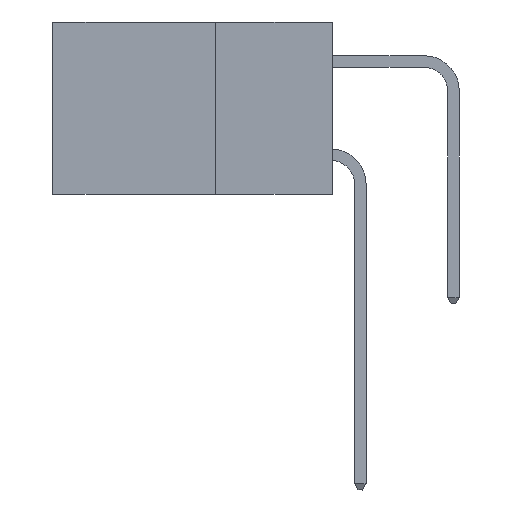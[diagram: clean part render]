
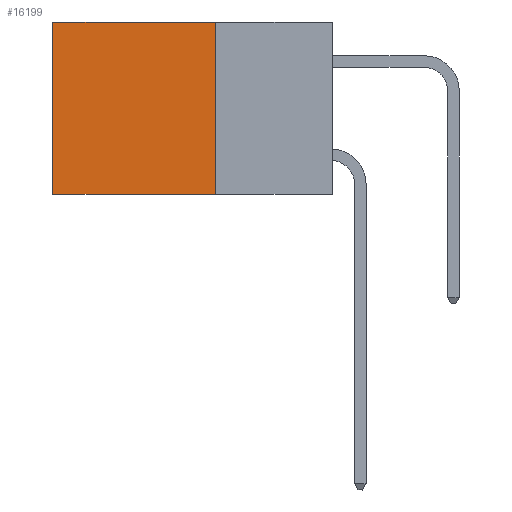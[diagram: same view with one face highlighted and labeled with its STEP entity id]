
A CAD part, left-side view. The second image highlights one B-rep face of the part: STEP entity #16199.
In plain terms, the highlighted planar face has unit normal (-1, 0, 0).
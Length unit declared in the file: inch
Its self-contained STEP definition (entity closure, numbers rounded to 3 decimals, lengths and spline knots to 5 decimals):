
#566 = EDGE_LOOP ( 'NONE', ( #21315, #25463, #12223, #2103 ) ) ;
#1255 = VERTEX_POINT ( 'NONE', #19544 ) ;
#1471 = CARTESIAN_POINT ( 'NONE',  ( 0.2615, 0.25, -0.37 ) ) ;
#1934 = VERTEX_POINT ( 'NONE', #1471 ) ;
#2103 = ORIENTED_EDGE ( 'NONE', *, *, #10400, .T. ) ;
#2178 = DIRECTION ( 'NONE',  ( 0., 0., -1. ) ) ;
#3205 = LINE ( 'NONE', #9441, #20774 ) ;
#3934 = DIRECTION ( 'NONE',  ( 1., 0., 0. ) ) ;
#3966 = CARTESIAN_POINT ( 'NONE',  ( 0.2615, 0.6, -0.37 ) ) ;
#4198 = CARTESIAN_POINT ( 'NONE',  ( 0.2615, 0.25, -0.37 ) ) ;
#4999 = VECTOR ( 'NONE', #22367, 39.37008 ) ;
#5414 = EDGE_CURVE ( 'NONE', #1934, #21194, #6059, .T. ) ;
#6059 = LINE ( 'NONE', #12390, #9311 ) ;
#9311 = VECTOR ( 'NONE', #16483, 39.37008 ) ;
#9441 = CARTESIAN_POINT ( 'NONE',  ( 0.2615, 0.25, -0.37 ) ) ;
#10400 = EDGE_CURVE ( 'NONE', #16912, #1255, #20462, .T. ) ;
#10540 = EDGE_CURVE ( 'NONE', #16912, #1934, #3205, .T. ) ;
#12223 = ORIENTED_EDGE ( 'NONE', *, *, #10540, .F. ) ;
#12390 = CARTESIAN_POINT ( 'NONE',  ( 0.2615, 0.25, -0.37 ) ) ;
#14495 = DIRECTION ( 'NONE',  ( 0., 1., 0. ) ) ;
#16199 = ADVANCED_FACE ( 'NONE', ( #22884 ), #20971, .F. ) ;
#16483 = DIRECTION ( 'NONE',  ( 0., 1., 0. ) ) ;
#16912 = VERTEX_POINT ( 'NONE', #19318 ) ;
#19318 = CARTESIAN_POINT ( 'NONE',  ( 0.2615, 0.25, 0. ) ) ;
#19468 = DIRECTION ( 'NONE',  ( 0., 0., -1. ) ) ;
#19544 = CARTESIAN_POINT ( 'NONE',  ( 0.2615, 0.6, 0. ) ) ;
#20462 = LINE ( 'NONE', #20741, #22910 ) ;
#20741 = CARTESIAN_POINT ( 'NONE',  ( 0.2615, 0.25, 0. ) ) ;
#20774 = VECTOR ( 'NONE', #19468, 39.37008 ) ;
#20971 = PLANE ( 'NONE',  #21048 ) ;
#21048 = AXIS2_PLACEMENT_3D ( 'NONE', #4198, #3934, #2178 ) ;
#21194 = VERTEX_POINT ( 'NONE', #21764 ) ;
#21315 = ORIENTED_EDGE ( 'NONE', *, *, #24093, .T. ) ;
#21764 = CARTESIAN_POINT ( 'NONE',  ( 0.2615, 0.6, -0.37 ) ) ;
#22367 = DIRECTION ( 'NONE',  ( 0., 0., -1. ) ) ;
#22516 = LINE ( 'NONE', #3966, #4999 ) ;
#22884 = FACE_OUTER_BOUND ( 'NONE', #566, .T. ) ;
#22910 = VECTOR ( 'NONE', #14495, 39.37008 ) ;
#24093 = EDGE_CURVE ( 'NONE', #1255, #21194, #22516, .T. ) ;
#25463 = ORIENTED_EDGE ( 'NONE', *, *, #5414, .F. ) ;
